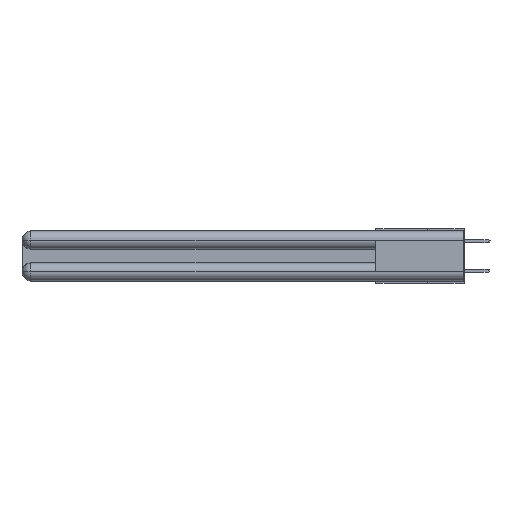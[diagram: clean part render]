
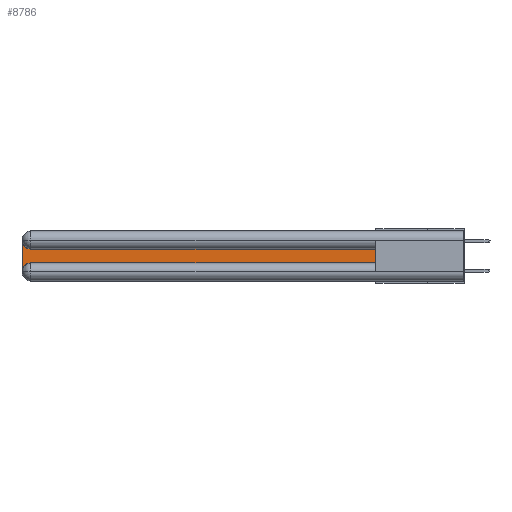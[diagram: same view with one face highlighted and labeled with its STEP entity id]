
A CAD part, left-side view. The second image highlights one B-rep face of the part: STEP entity #8786.
In plain terms, the highlighted planar face has unit normal (-1, 0, 0).
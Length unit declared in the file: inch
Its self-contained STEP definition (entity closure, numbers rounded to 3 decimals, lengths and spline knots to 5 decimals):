
#144 = ORIENTED_EDGE ( 'NONE', *, *, #26383, .T. ) ;
#306 = LINE ( 'NONE', #23560, #33530 ) ;
#1799 = CARTESIAN_POINT ( 'NONE',  ( 0.075, 0.6, -0.1225 ) ) ;
#1917 = DIRECTION ( 'NONE',  ( 0., -1., 0. ) ) ;
#2329 = AXIS2_PLACEMENT_3D ( 'NONE', #29252, #26516, #26292 ) ;
#2953 = FACE_OUTER_BOUND ( 'NONE', #16726, .T. ) ;
#3539 = EDGE_CURVE ( 'NONE', #33041, #23756, #10207, .T. ) ;
#3584 = EDGE_CURVE ( 'NONE', #4180, #23850, #16803, .T. ) ;
#4180 = VERTEX_POINT ( 'NONE', #19691 ) ;
#4430 = VECTOR ( 'NONE', #25423, 39.37008 ) ;
#5339 = LINE ( 'NONE', #16466, #18051 ) ;
#8183 = ORIENTED_EDGE ( 'NONE', *, *, #20578, .T. ) ;
#8379 = CARTESIAN_POINT ( 'NONE',  ( 0.075, 2.94, -0.2775 ) ) ;
#8786 = ADVANCED_FACE ( 'NONE', ( #2953 ), #28548, .F. ) ;
#9220 = EDGE_CURVE ( 'NONE', #23662, #4180, #17303, .T. ) ;
#10207 = LINE ( 'NONE', #1799, #4430 ) ;
#11859 = EDGE_CURVE ( 'NONE', #22595, #23662, #5339, .T. ) ;
#13296 = CIRCLE ( 'NONE', #2329, 0.06 ) ;
#13674 = DIRECTION ( 'NONE',  ( 0., 0., -1. ) ) ;
#15085 = CARTESIAN_POINT ( 'NONE',  ( 0.075, 3., -0.0625 ) ) ;
#15552 = CARTESIAN_POINT ( 'NONE',  ( 0.075, 3., -0.1225 ) ) ;
#16466 = CARTESIAN_POINT ( 'NONE',  ( 0.075, 3., -0.2175 ) ) ;
#16665 = DIRECTION ( 'NONE',  ( 1., 0., 0. ) ) ;
#16726 = EDGE_LOOP ( 'NONE', ( #21692, #8183, #33452, #18120, #29921, #144 ) ) ;
#16803 = LINE ( 'NONE', #23011, #25344 ) ;
#17303 = CIRCLE ( 'NONE', #29125, 0.06 ) ;
#18051 = VECTOR ( 'NONE', #25107, 39.37008 ) ;
#18120 = ORIENTED_EDGE ( 'NONE', *, *, #9220, .T. ) ;
#18164 = DIRECTION ( 'NONE',  ( 1., 0., 0. ) ) ;
#19691 = CARTESIAN_POINT ( 'NONE',  ( 0.075, 2.94, -0.2175 ) ) ;
#19707 = AXIS2_PLACEMENT_3D ( 'NONE', #15552, #18164, #23419 ) ;
#20578 = EDGE_CURVE ( 'NONE', #23756, #22595, #13296, .T. ) ;
#21692 = ORIENTED_EDGE ( 'NONE', *, *, #3539, .T. ) ;
#22595 = VERTEX_POINT ( 'NONE', #15085 ) ;
#23011 = CARTESIAN_POINT ( 'NONE',  ( 0.075, 0.6, -0.2175 ) ) ;
#23419 = DIRECTION ( 'NONE',  ( 0., 0., -1. ) ) ;
#23560 = CARTESIAN_POINT ( 'NONE',  ( 0.075, 0.6, -0.2175 ) ) ;
#23662 = VERTEX_POINT ( 'NONE', #26502 ) ;
#23756 = VERTEX_POINT ( 'NONE', #26835 ) ;
#23850 = VERTEX_POINT ( 'NONE', #29348 ) ;
#25107 = DIRECTION ( 'NONE',  ( 0., 0., -1. ) ) ;
#25344 = VECTOR ( 'NONE', #1917, 39.37008 ) ;
#25423 = DIRECTION ( 'NONE',  ( 0., 1., 0. ) ) ;
#26292 = DIRECTION ( 'NONE',  ( 0., 0., -1. ) ) ;
#26383 = EDGE_CURVE ( 'NONE', #23850, #33041, #306, .T. ) ;
#26502 = CARTESIAN_POINT ( 'NONE',  ( 0.075, 3., -0.2775 ) ) ;
#26516 = DIRECTION ( 'NONE',  ( 1., 0., 0. ) ) ;
#26835 = CARTESIAN_POINT ( 'NONE',  ( 0.075, 2.94, -0.1225 ) ) ;
#28548 = PLANE ( 'NONE',  #19707 ) ;
#28931 = DIRECTION ( 'NONE',  ( 0., 0., 1. ) ) ;
#29125 = AXIS2_PLACEMENT_3D ( 'NONE', #8379, #16665, #13674 ) ;
#29252 = CARTESIAN_POINT ( 'NONE',  ( 0.075, 2.94, -0.0625 ) ) ;
#29348 = CARTESIAN_POINT ( 'NONE',  ( 0.075, 0.6, -0.2175 ) ) ;
#29921 = ORIENTED_EDGE ( 'NONE', *, *, #3584, .T. ) ;
#30470 = CARTESIAN_POINT ( 'NONE',  ( 0.075, 0.6, -0.1225 ) ) ;
#33041 = VERTEX_POINT ( 'NONE', #30470 ) ;
#33452 = ORIENTED_EDGE ( 'NONE', *, *, #11859, .T. ) ;
#33530 = VECTOR ( 'NONE', #28931, 39.37008 ) ;
